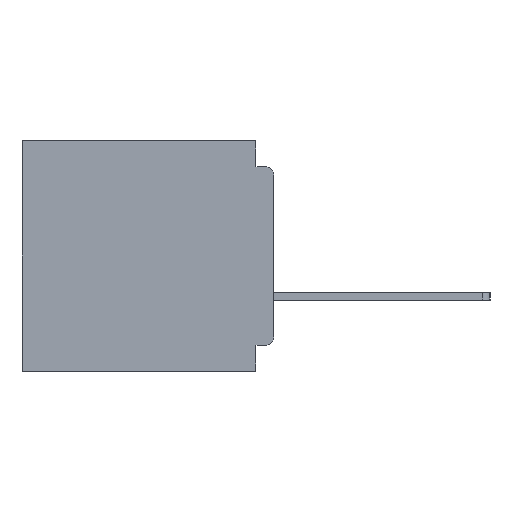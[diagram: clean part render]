
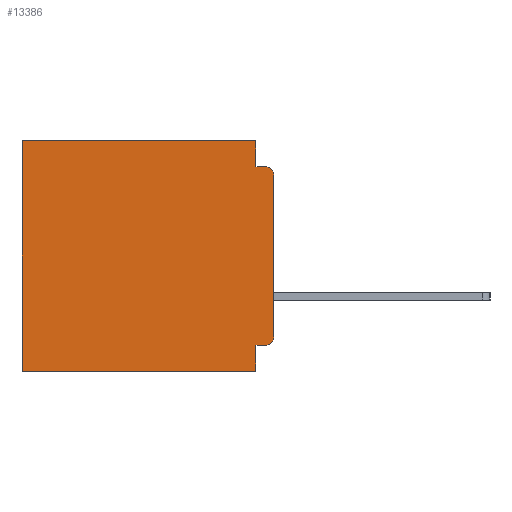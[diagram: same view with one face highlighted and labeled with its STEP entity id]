
A CAD part, left-side view. The second image highlights one B-rep face of the part: STEP entity #13386.
In plain terms, the highlighted planar face has unit normal (-1, 0, 0).
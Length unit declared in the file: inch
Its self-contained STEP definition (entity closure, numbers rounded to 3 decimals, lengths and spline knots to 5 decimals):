
#421 = CARTESIAN_POINT ( 'NONE',  ( 0.3, 0.437, -0.4 ) ) ;
#496 = VECTOR ( 'NONE', #18394, 39.37008 ) ;
#983 = EDGE_CURVE ( 'NONE', #51430, #30364, #6731, .T. ) ;
#1546 = CARTESIAN_POINT ( 'NONE',  ( 0.3, 0.031, -0.4 ) ) ;
#4593 = DIRECTION ( 'NONE',  ( 0., 1., 0. ) ) ;
#5503 = DIRECTION ( 'NONE',  ( 0., 1., 0. ) ) ;
#5635 = EDGE_CURVE ( 'NONE', #18821, #29712, #20923, .T. ) ;
#6601 = DIRECTION ( 'NONE',  ( 0., 0., -1. ) ) ;
#6711 = EDGE_CURVE ( 'NONE', #11272, #29712, #49592, .T. ) ;
#6731 = LINE ( 'NONE', #45822, #31281 ) ;
#7090 = EDGE_CURVE ( 'NONE', #17583, #43560, #15786, .T. ) ;
#7206 = DIRECTION ( 'NONE',  ( -1., 0., 0. ) ) ;
#7321 = CARTESIAN_POINT ( 'NONE',  ( 0.3, 0.031, 0. ) ) ;
#8643 = LINE ( 'NONE', #23028, #43865 ) ;
#9009 = ORIENTED_EDGE ( 'NONE', *, *, #6711, .F. ) ;
#11272 = VERTEX_POINT ( 'NONE', #44547 ) ;
#11556 = VECTOR ( 'NONE', #32860, 39.37008 ) ;
#11770 = EDGE_LOOP ( 'NONE', ( #37827, #22738, #35387, #56413, #29897, #17652, #9009, #50948, #54887, #21333 ) ) ;
#11940 = CARTESIAN_POINT ( 'NONE',  ( 0.3, 0., -0.045 ) ) ;
#13386 = ADVANCED_FACE ( 'NONE', ( #21943 ), #34028, .F. ) ;
#14911 = AXIS2_PLACEMENT_3D ( 'NONE', #15953, #48064, #20586 ) ;
#15388 = EDGE_CURVE ( 'NONE', #51430, #55459, #19763, .T. ) ;
#15786 = LINE ( 'NONE', #7321, #38805 ) ;
#15953 = CARTESIAN_POINT ( 'NONE',  ( 0.3, 0.015, -0.34 ) ) ;
#17583 = VERTEX_POINT ( 'NONE', #26481 ) ;
#17652 = ORIENTED_EDGE ( 'NONE', *, *, #5635, .T. ) ;
#18394 = DIRECTION ( 'NONE',  ( 0., 1., 0. ) ) ;
#18821 = VERTEX_POINT ( 'NONE', #30583 ) ;
#19763 = CIRCLE ( 'NONE', #51912, 0.015 ) ;
#20586 = DIRECTION ( 'NONE',  ( 0., 0., -1. ) ) ;
#20923 = LINE ( 'NONE', #421, #11556 ) ;
#21333 = ORIENTED_EDGE ( 'NONE', *, *, #38114, .T. ) ;
#21943 = FACE_OUTER_BOUND ( 'NONE', #11770, .T. ) ;
#22738 = ORIENTED_EDGE ( 'NONE', *, *, #15388, .T. ) ;
#23028 = CARTESIAN_POINT ( 'NONE',  ( 0.3, 0., -0.355 ) ) ;
#26481 = CARTESIAN_POINT ( 'NONE',  ( 0.3, 0.031, 0. ) ) ;
#28496 = CARTESIAN_POINT ( 'NONE',  ( 0.3, 0., 0. ) ) ;
#28889 = CARTESIAN_POINT ( 'NONE',  ( 0.3, 0., -0.06 ) ) ;
#29712 = VERTEX_POINT ( 'NONE', #49518 ) ;
#29897 = ORIENTED_EDGE ( 'NONE', *, *, #34593, .T. ) ;
#30364 = VERTEX_POINT ( 'NONE', #32861 ) ;
#30583 = CARTESIAN_POINT ( 'NONE',  ( 0.3, 0.437, 0. ) ) ;
#31281 = VECTOR ( 'NONE', #44051, 39.37008 ) ;
#32860 = DIRECTION ( 'NONE',  ( 0., 0., -1. ) ) ;
#32861 = CARTESIAN_POINT ( 'NONE',  ( 0.3, 0., -0.34 ) ) ;
#32960 = EDGE_CURVE ( 'NONE', #43490, #11272, #36037, .T. ) ;
#34028 = PLANE ( 'NONE',  #40389 ) ;
#34210 = DIRECTION ( 'NONE',  ( 1., 0., 0. ) ) ;
#34593 = EDGE_CURVE ( 'NONE', #17583, #18821, #38047, .T. ) ;
#34626 = VECTOR ( 'NONE', #43146, 39.37008 ) ;
#34803 = CARTESIAN_POINT ( 'NONE',  ( 0.3, 0.015, -0.06 ) ) ;
#35092 = DIRECTION ( 'NONE',  ( 0., 0., -1. ) ) ;
#35387 = ORIENTED_EDGE ( 'NONE', *, *, #53868, .F. ) ;
#36037 = LINE ( 'NONE', #1546, #34626 ) ;
#36119 = CARTESIAN_POINT ( 'NONE',  ( 0.3, 0.015, -0.355 ) ) ;
#36622 = VECTOR ( 'NONE', #5503, 39.37008 ) ;
#37827 = ORIENTED_EDGE ( 'NONE', *, *, #983, .F. ) ;
#38047 = LINE ( 'NONE', #28496, #36622 ) ;
#38114 = EDGE_CURVE ( 'NONE', #39798, #30364, #44890, .T. ) ;
#38805 = VECTOR ( 'NONE', #35092, 39.37008 ) ;
#39385 = DIRECTION ( 'NONE',  ( 0., 0., -1. ) ) ;
#39454 = DIRECTION ( 'NONE',  ( 0., -1., 0. ) ) ;
#39798 = VERTEX_POINT ( 'NONE', #36119 ) ;
#40389 = AXIS2_PLACEMENT_3D ( 'NONE', #43196, #34210, #6601 ) ;
#43146 = DIRECTION ( 'NONE',  ( 0., 0., -1. ) ) ;
#43196 = CARTESIAN_POINT ( 'NONE',  ( 0.3, 0., -0.4 ) ) ;
#43490 = VERTEX_POINT ( 'NONE', #43872 ) ;
#43560 = VERTEX_POINT ( 'NONE', #49262 ) ;
#43865 = VECTOR ( 'NONE', #4593, 39.37008 ) ;
#43872 = CARTESIAN_POINT ( 'NONE',  ( 0.3, 0.031, -0.355 ) ) ;
#44051 = DIRECTION ( 'NONE',  ( 0., 0., -1. ) ) ;
#44547 = CARTESIAN_POINT ( 'NONE',  ( 0.3, 0.031, -0.4 ) ) ;
#44890 = CIRCLE ( 'NONE', #14911, 0.015 ) ;
#45050 = EDGE_CURVE ( 'NONE', #39798, #43490, #8643, .T. ) ;
#45642 = VECTOR ( 'NONE', #39454, 39.37008 ) ;
#45822 = CARTESIAN_POINT ( 'NONE',  ( 0.3, 0., -0.4 ) ) ;
#48064 = DIRECTION ( 'NONE',  ( -1., 0., 0. ) ) ;
#49262 = CARTESIAN_POINT ( 'NONE',  ( 0.3, 0.031, -0.045 ) ) ;
#49518 = CARTESIAN_POINT ( 'NONE',  ( 0.3, 0.437, -0.4 ) ) ;
#49592 = LINE ( 'NONE', #50539, #496 ) ;
#50539 = CARTESIAN_POINT ( 'NONE',  ( 0.3, 0., -0.4 ) ) ;
#50948 = ORIENTED_EDGE ( 'NONE', *, *, #32960, .F. ) ;
#51430 = VERTEX_POINT ( 'NONE', #28889 ) ;
#51667 = CARTESIAN_POINT ( 'NONE',  ( 0.3, 0.015, -0.045 ) ) ;
#51912 = AXIS2_PLACEMENT_3D ( 'NONE', #34803, #7206, #39385 ) ;
#53868 = EDGE_CURVE ( 'NONE', #43560, #55459, #59138, .T. ) ;
#54887 = ORIENTED_EDGE ( 'NONE', *, *, #45050, .F. ) ;
#55459 = VERTEX_POINT ( 'NONE', #51667 ) ;
#56413 = ORIENTED_EDGE ( 'NONE', *, *, #7090, .F. ) ;
#59138 = LINE ( 'NONE', #11940, #45642 ) ;
